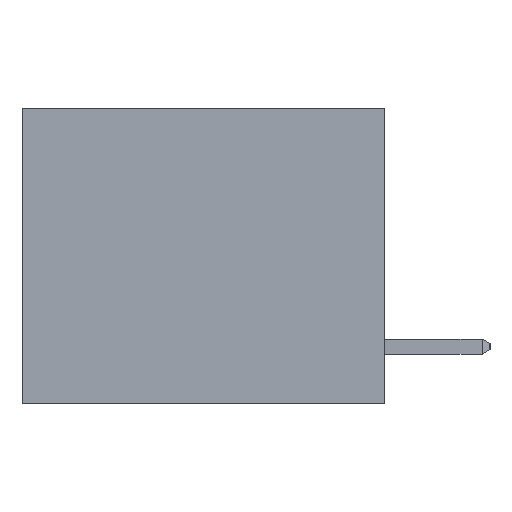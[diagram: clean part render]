
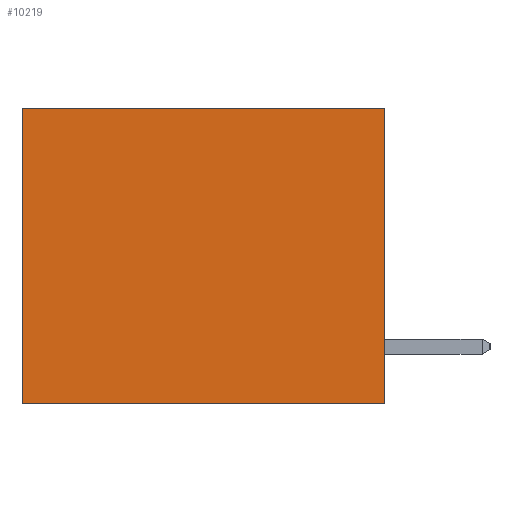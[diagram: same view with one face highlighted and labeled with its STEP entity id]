
A CAD part, left-side view. The second image highlights one B-rep face of the part: STEP entity #10219.
In plain terms, the highlighted planar face has unit normal (-1, 0, 0).
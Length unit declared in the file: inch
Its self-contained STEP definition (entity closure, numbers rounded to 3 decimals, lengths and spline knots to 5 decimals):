
#101 = EDGE_CURVE ( 'NONE', #2814, #10165, #11399, .T. ) ;
#431 = DIRECTION ( 'NONE',  ( 0., 1., 0. ) ) ;
#691 = ORIENTED_EDGE ( 'NONE', *, *, #9980, .T. ) ;
#800 = EDGE_CURVE ( 'NONE', #10165, #10481, #10810, .T. ) ;
#953 = AXIS2_PLACEMENT_3D ( 'NONE', #5321, #4397, #6211 ) ;
#2485 = FACE_OUTER_BOUND ( 'NONE', #5614, .T. ) ;
#2814 = VERTEX_POINT ( 'NONE', #11183 ) ;
#3467 = ORIENTED_EDGE ( 'NONE', *, *, #6600, .T. ) ;
#3599 = LINE ( 'NONE', #6947, #10623 ) ;
#4397 = DIRECTION ( 'NONE',  ( 1., 0., 0. ) ) ;
#4553 = CARTESIAN_POINT ( 'NONE',  ( 0.3165, 0.6, -0.49 ) ) ;
#5321 = CARTESIAN_POINT ( 'NONE',  ( 0.3165, 0., -0.49 ) ) ;
#5614 = EDGE_LOOP ( 'NONE', ( #691, #11657, #11327, #3467 ) ) ;
#5872 = CARTESIAN_POINT ( 'NONE',  ( 0.3165, 0.6, 0. ) ) ;
#6044 = CARTESIAN_POINT ( 'NONE',  ( 0.3165, 0., -0.49 ) ) ;
#6135 = PLANE ( 'NONE',  #953 ) ;
#6160 = CARTESIAN_POINT ( 'NONE',  ( 0.3165, 0., -0.49 ) ) ;
#6211 = DIRECTION ( 'NONE',  ( 0., 0., -1. ) ) ;
#6600 = EDGE_CURVE ( 'NONE', #2814, #8708, #3599, .T. ) ;
#6947 = CARTESIAN_POINT ( 'NONE',  ( 0.3165, 0., 0. ) ) ;
#7425 = VECTOR ( 'NONE', #8281, 39.37008 ) ;
#7986 = DIRECTION ( 'NONE',  ( 0., 0., -1. ) ) ;
#8281 = DIRECTION ( 'NONE',  ( 0., 0., -1. ) ) ;
#8708 = VERTEX_POINT ( 'NONE', #5872 ) ;
#8949 = VECTOR ( 'NONE', #10906, 39.37008 ) ;
#8966 = VECTOR ( 'NONE', #7986, 39.37008 ) ;
#8970 = CARTESIAN_POINT ( 'NONE',  ( 0.3165, 0.6, -0.49 ) ) ;
#9840 = LINE ( 'NONE', #4553, #7425 ) ;
#9980 = EDGE_CURVE ( 'NONE', #8708, #10481, #9840, .T. ) ;
#10165 = VERTEX_POINT ( 'NONE', #10756 ) ;
#10219 = ADVANCED_FACE ( 'NONE', ( #2485 ), #6135, .F. ) ;
#10481 = VERTEX_POINT ( 'NONE', #8970 ) ;
#10623 = VECTOR ( 'NONE', #431, 39.37008 ) ;
#10756 = CARTESIAN_POINT ( 'NONE',  ( 0.3165, 0., -0.49 ) ) ;
#10810 = LINE ( 'NONE', #6044, #8949 ) ;
#10906 = DIRECTION ( 'NONE',  ( 0., 1., 0. ) ) ;
#11183 = CARTESIAN_POINT ( 'NONE',  ( 0.3165, 0., 0. ) ) ;
#11327 = ORIENTED_EDGE ( 'NONE', *, *, #101, .F. ) ;
#11399 = LINE ( 'NONE', #6160, #8966 ) ;
#11657 = ORIENTED_EDGE ( 'NONE', *, *, #800, .F. ) ;
